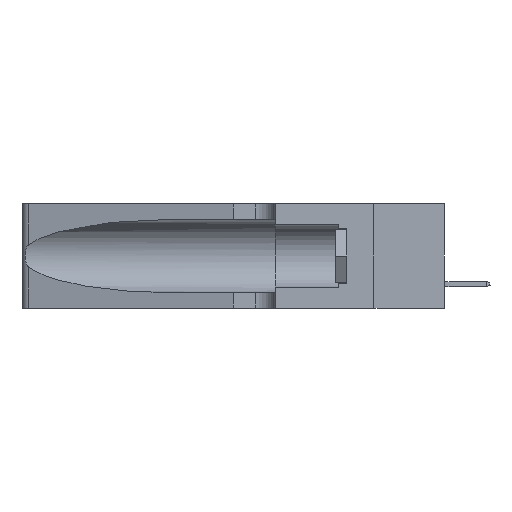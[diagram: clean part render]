
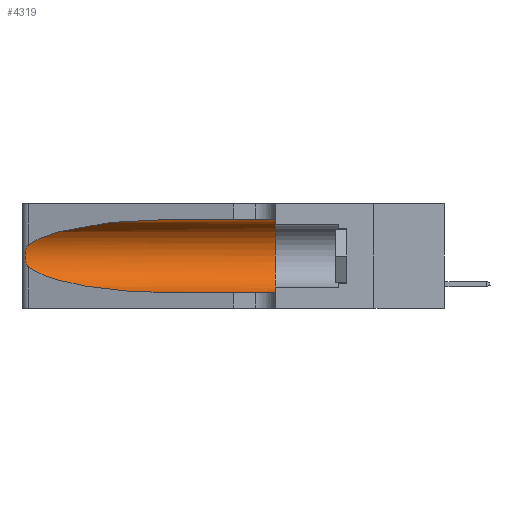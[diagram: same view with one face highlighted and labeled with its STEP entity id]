
A CAD part, left-side view. The second image highlights one B-rep face of the part: STEP entity #4319.
In plain terms, the highlighted cylindrical face has radius 3.308 mm (diameter 6.617 mm), a partial arc.
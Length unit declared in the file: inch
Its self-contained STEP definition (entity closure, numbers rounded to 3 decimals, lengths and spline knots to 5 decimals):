
#92 = AXIS2_PLACEMENT_3D ( 'NONE', #32011, #8611, #26824 ) ;
#2340 = B_SPLINE_CURVE_WITH_KNOTS ( 'NONE', 3,
 ( #7688, #26126, #15417, #5378, #26238, #33718, #13141, #33837, #18490, #10648, #31068, #10417, #23293, #18376 ),
 .UNSPECIFIED., .F., .F.,
 ( 4, 2, 2, 2, 2, 2, 4 ),
 ( 0., 0.00027, 0.00053, 0.00107, 0.0016, 0.00187, 0.00214 ),
 .UNSPECIFIED. ) ;
#2626 = CARTESIAN_POINT ( 'NONE',  ( 0.25487, 1.22718, 0.14631 ) ) ;
#2757 = ORIENTED_EDGE ( 'NONE', *, *, #32168, .T. ) ;
#3143 = CARTESIAN_POINT ( 'NONE',  ( 0.25487, 1.22718, 0.14631 ) ) ;
#3369 = EDGE_CURVE ( 'NONE', #25662, #29019, #26152, .T. ) ;
#3377 =( BOUNDED_CURVE ( )  B_SPLINE_CURVE ( 3, ( #10944, #13345, #16170, #13462 ),
 .UNSPECIFIED., .F., .F. ) 
 B_SPLINE_CURVE_WITH_KNOTS ( ( 4, 4 ),
 ( 1.5708, 2.84003 ),
 .UNSPECIFIED. ) 
 CURVE ( )  GEOMETRIC_REPRESENTATION_ITEM ( )  RATIONAL_B_SPLINE_CURVE ( ( 1., 0.87, 0.87, 1. ) ) 
 REPRESENTATION_ITEM ( '' )  );
#4319 = ADVANCED_FACE ( 'NONE', ( #16731 ), #7751, .F. ) ;
#4678 = ORIENTED_EDGE ( 'NONE', *, *, #31088, .T. ) ;
#4925 = DIRECTION ( 'NONE',  ( 0., -1., 0. ) ) ;
#5378 = CARTESIAN_POINT ( 'NONE',  ( 0.25787, 1.23484, 0.2124 ) ) ;
#5933 = VERTEX_POINT ( 'NONE', #25918 ) ;
#7688 = CARTESIAN_POINT ( 'NONE',  ( 0.25487, 1.22718, 0.22369 ) ) ;
#7751 = CYLINDRICAL_SURFACE ( 'NONE', #27713, 0.13025 ) ;
#8611 = DIRECTION ( 'NONE',  ( 0., 1., 0. ) ) ;
#8909 = CARTESIAN_POINT ( 'NONE',  ( 0.1305, 0.72297, 0.31525 ) ) ;
#9209 = CARTESIAN_POINT ( 'NONE',  ( 0.18966, 0.96281, 0.05475 ) ) ;
#10417 = CARTESIAN_POINT ( 'NONE',  ( 0.25639, 1.23186, 0.15144 ) ) ;
#10648 = CARTESIAN_POINT ( 'NONE',  ( 0.25856, 1.23593, 0.16098 ) ) ;
#10718 = LINE ( 'NONE', #16216, #14381 ) ;
#10944 = CARTESIAN_POINT ( 'NONE',  ( 0.1305, 0.72297, 0.31525 ) ) ;
#11070 = ORIENTED_EDGE ( 'NONE', *, *, #3369, .F. ) ;
#12765 = VERTEX_POINT ( 'NONE', #2626 ) ;
#13141 = CARTESIAN_POINT ( 'NONE',  ( 0.26075, 1.23896, 0.19203 ) ) ;
#13345 = CARTESIAN_POINT ( 'NONE',  ( 0.18966, 0.96281, 0.31525 ) ) ;
#13462 = CARTESIAN_POINT ( 'NONE',  ( 0.25487, 1.22718, 0.22369 ) ) ;
#13638 = CARTESIAN_POINT ( 'NONE',  ( 0.2373, 1.15595, 0.08982 ) ) ;
#14381 = VECTOR ( 'NONE', #26706, 39.37008 ) ;
#14540 = DIRECTION ( 'NONE',  ( 0., -1., 0. ) ) ;
#15417 = CARTESIAN_POINT ( 'NONE',  ( 0.25639, 1.23184, 0.21858 ) ) ;
#15481 = CARTESIAN_POINT ( 'NONE',  ( 0.1305, 0.72297, 0.05475 ) ) ;
#16170 = CARTESIAN_POINT ( 'NONE',  ( 0.2373, 1.15595, 0.28018 ) ) ;
#16205 = VERTEX_POINT ( 'NONE', #8909 ) ;
#16216 = CARTESIAN_POINT ( 'NONE',  ( 0.1305, 1.61858, 0.05475 ) ) ;
#16731 = FACE_OUTER_BOUND ( 'NONE', #29211, .T. ) ;
#17033 = CARTESIAN_POINT ( 'NONE',  ( 0.1305, 0.35, 0.05475 ) ) ;
#17047 = CARTESIAN_POINT ( 'NONE',  ( 0.1305, 1.61858, 0.185 ) ) ;
#18376 = CARTESIAN_POINT ( 'NONE',  ( 0.25487, 1.22718, 0.14631 ) ) ;
#18490 = CARTESIAN_POINT ( 'NONE',  ( 0.26017, 1.23833, 0.17102 ) ) ;
#18661 = ORIENTED_EDGE ( 'NONE', *, *, #21589, .T. ) ;
#20344 = VERTEX_POINT ( 'NONE', #15481 ) ;
#21589 = EDGE_CURVE ( 'NONE', #20344, #29019, #10718, .T. ) ;
#22343 = EDGE_CURVE ( 'NONE', #12765, #20344, #24494, .T. ) ;
#22429 = DIRECTION ( 'NONE',  ( 0., 0., -1. ) ) ;
#22625 = EDGE_CURVE ( 'NONE', #16205, #25662, #26171, .T. ) ;
#23293 = CARTESIAN_POINT ( 'NONE',  ( 0.25555, 1.22993, 0.14849 ) ) ;
#24494 =( BOUNDED_CURVE ( )  B_SPLINE_CURVE ( 3, ( #3143, #13638, #9209, #24683 ),
 .UNSPECIFIED., .F., .T. ) 
 B_SPLINE_CURVE_WITH_KNOTS ( ( 4, 4 ),
 ( 3.44316, 4.71239 ),
 .UNSPECIFIED. ) 
 CURVE ( )  GEOMETRIC_REPRESENTATION_ITEM ( )  RATIONAL_B_SPLINE_CURVE ( ( 1., 0.87, 0.87, 1. ) ) 
 REPRESENTATION_ITEM ( '' )  );
#24683 = CARTESIAN_POINT ( 'NONE',  ( 0.1305, 0.72297, 0.05475 ) ) ;
#25579 = CARTESIAN_POINT ( 'NONE',  ( 0.1305, 1.61858, 0.31525 ) ) ;
#25662 = VERTEX_POINT ( 'NONE', #31270 ) ;
#25918 = CARTESIAN_POINT ( 'NONE',  ( 0.25487, 1.22718, 0.22369 ) ) ;
#26126 = CARTESIAN_POINT ( 'NONE',  ( 0.25555, 1.22994, 0.2215 ) ) ;
#26152 = CIRCLE ( 'NONE', #92, 0.13025 ) ;
#26171 = LINE ( 'NONE', #25579, #28230 ) ;
#26238 = CARTESIAN_POINT ( 'NONE',  ( 0.25854, 1.2359, 0.20912 ) ) ;
#26706 = DIRECTION ( 'NONE',  ( 0., -1., 0. ) ) ;
#26824 = DIRECTION ( 'NONE',  ( 0., 0., 1. ) ) ;
#27119 = ORIENTED_EDGE ( 'NONE', *, *, #22625, .F. ) ;
#27713 = AXIS2_PLACEMENT_3D ( 'NONE', #17047, #14540, #22429 ) ;
#28230 = VECTOR ( 'NONE', #4925, 39.37008 ) ;
#29019 = VERTEX_POINT ( 'NONE', #17033 ) ;
#29211 = EDGE_LOOP ( 'NONE', ( #4678, #2757, #31239, #18661, #11070, #27119 ) ) ;
#31068 = CARTESIAN_POINT ( 'NONE',  ( 0.25789, 1.23486, 0.15765 ) ) ;
#31088 = EDGE_CURVE ( 'NONE', #16205, #5933, #3377, .T. ) ;
#31239 = ORIENTED_EDGE ( 'NONE', *, *, #22343, .T. ) ;
#31270 = CARTESIAN_POINT ( 'NONE',  ( 0.1305, 0.35, 0.31525 ) ) ;
#32011 = CARTESIAN_POINT ( 'NONE',  ( 0.1305, 0.35, 0.185 ) ) ;
#32168 = EDGE_CURVE ( 'NONE', #5933, #12765, #2340, .T. ) ;
#33718 = CARTESIAN_POINT ( 'NONE',  ( 0.26018, 1.23835, 0.19895 ) ) ;
#33837 = CARTESIAN_POINT ( 'NONE',  ( 0.26075, 1.23896, 0.178 ) ) ;
